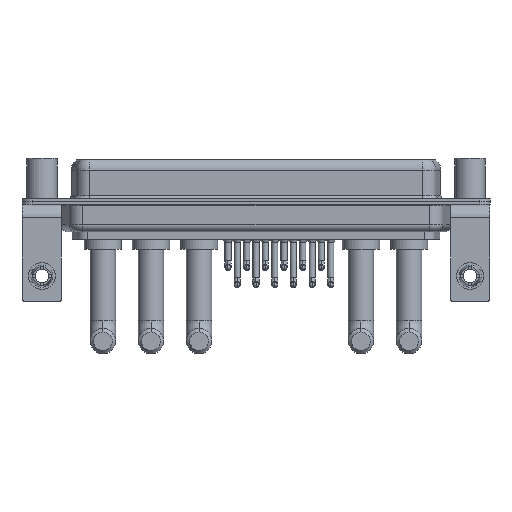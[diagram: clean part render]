
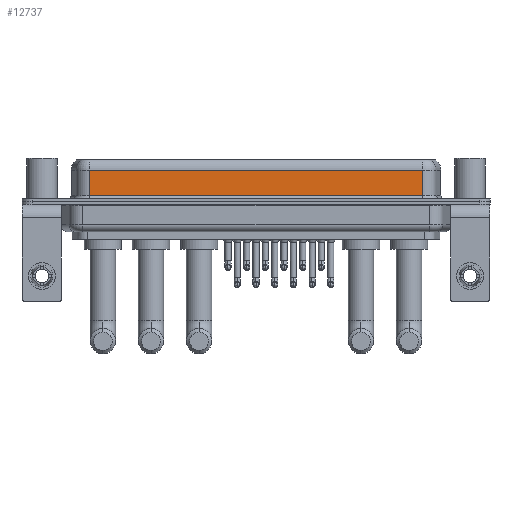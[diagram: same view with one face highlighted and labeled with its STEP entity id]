
A CAD part, front view. The second image highlights one B-rep face of the part: STEP entity #12737.
In plain terms, the highlighted planar face has unit normal (0, -1, 0).
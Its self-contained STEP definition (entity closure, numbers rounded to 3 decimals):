
#518 = ORIENTED_EDGE ( 'NONE', *, *, #15074, .T. ) ;
#4074 = CARTESIAN_POINT ( 'NONE',  ( 56.462, -3.95, 0.9 ) ) ;
#4309 = DIRECTION ( 'NONE',  ( 1., 0., 0. ) ) ;
#4836 = VECTOR ( 'NONE', #20900, 1000. ) ;
#4969 = PLANE ( 'NONE',  #21282 ) ;
#5394 = CARTESIAN_POINT ( 'NONE',  ( 56.462, -3.95, 6.4 ) ) ;
#5440 = VERTEX_POINT ( 'NONE', #20684 ) ;
#5540 = VECTOR ( 'NONE', #20165, 1000. ) ;
#5865 = CARTESIAN_POINT ( 'NONE',  ( 56.462, -3.95, 4.65 ) ) ;
#7341 = CARTESIAN_POINT ( 'NONE',  ( 7.038, -3.95, 4.65 ) ) ;
#9919 = LINE ( 'NONE', #4074, #13680 ) ;
#10270 = CARTESIAN_POINT ( 'NONE',  ( 56.462, -3.95, 0.9 ) ) ;
#10606 = CARTESIAN_POINT ( 'NONE',  ( 56.462, -3.95, 6.4 ) ) ;
#11245 = EDGE_LOOP ( 'NONE', ( #22559, #518, #21215, #19176 ) ) ;
#11780 = VERTEX_POINT ( 'NONE', #10270 ) ;
#12183 = DIRECTION ( 'NONE',  ( 0., 0., 1. ) ) ;
#12737 = ADVANCED_FACE ( 'NONE', ( #17979 ), #4969, .F. ) ;
#13201 = LINE ( 'NONE', #5865, #4836 ) ;
#13680 = VECTOR ( 'NONE', #4309, 1000. ) ;
#15022 = EDGE_CURVE ( 'NONE', #18571, #11780, #21878, .T. ) ;
#15074 = EDGE_CURVE ( 'NONE', #18571, #22543, #13201, .T. ) ;
#16179 = DIRECTION ( 'NONE',  ( 0., 1., 0. ) ) ;
#16553 = EDGE_CURVE ( 'NONE', #5440, #11780, #9919, .T. ) ;
#17979 = FACE_OUTER_BOUND ( 'NONE', #11245, .T. ) ;
#18237 = LINE ( 'NONE', #19937, #5540 ) ;
#18571 = VERTEX_POINT ( 'NONE', #19801 ) ;
#19176 = ORIENTED_EDGE ( 'NONE', *, *, #16553, .T. ) ;
#19584 = EDGE_CURVE ( 'NONE', #22543, #5440, #18237, .T. ) ;
#19801 = CARTESIAN_POINT ( 'NONE',  ( 56.462, -3.95, 4.65 ) ) ;
#19937 = CARTESIAN_POINT ( 'NONE',  ( 7.038, -3.95, 6.4 ) ) ;
#20165 = DIRECTION ( 'NONE',  ( 0., 0., -1. ) ) ;
#20327 = DIRECTION ( 'NONE',  ( 0., 0., -1. ) ) ;
#20684 = CARTESIAN_POINT ( 'NONE',  ( 7.038, -3.95, 0.9 ) ) ;
#20900 = DIRECTION ( 'NONE',  ( -1., 0., 0. ) ) ;
#21215 = ORIENTED_EDGE ( 'NONE', *, *, #19584, .T. ) ;
#21282 = AXIS2_PLACEMENT_3D ( 'NONE', #10606, #16179, #12183 ) ;
#21374 = VECTOR ( 'NONE', #20327, 1000. ) ;
#21878 = LINE ( 'NONE', #5394, #21374 ) ;
#22543 = VERTEX_POINT ( 'NONE', #7341 ) ;
#22559 = ORIENTED_EDGE ( 'NONE', *, *, #15022, .F. ) ;
